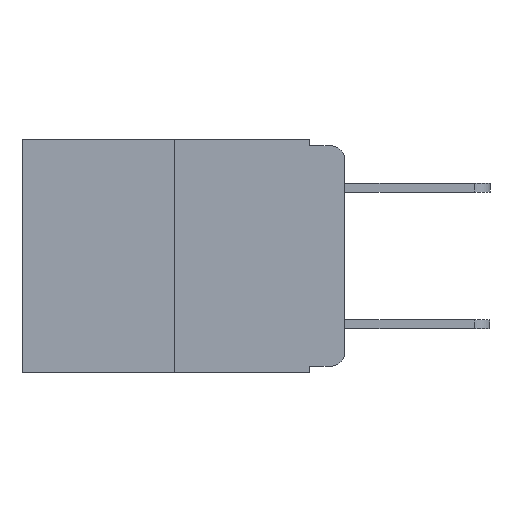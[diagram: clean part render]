
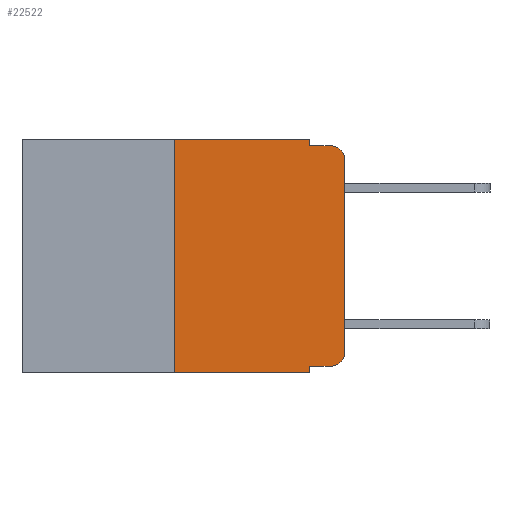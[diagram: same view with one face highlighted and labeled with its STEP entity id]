
A CAD part, left-side view. The second image highlights one B-rep face of the part: STEP entity #22522.
In plain terms, the highlighted planar face has unit normal (-1, 0, 0).
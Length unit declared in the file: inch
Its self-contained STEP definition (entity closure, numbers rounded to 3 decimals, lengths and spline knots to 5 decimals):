
#40 = ORIENTED_EDGE ( 'NONE', *, *, #12396, .T. ) ;
#79 = ORIENTED_EDGE ( 'NONE', *, *, #18576, .F. ) ;
#136 = DIRECTION ( 'NONE',  ( 0., 0., -1. ) ) ;
#841 = CIRCLE ( 'NONE', #1884, 0.02 ) ;
#1027 = ORIENTED_EDGE ( 'NONE', *, *, #13814, .F. ) ;
#1268 = CARTESIAN_POINT ( 'NONE',  ( 0., 0.25, -0.343 ) ) ;
#1884 = AXIS2_PLACEMENT_3D ( 'NONE', #23375, #11987, #136 ) ;
#2497 = DIRECTION ( 'NONE',  ( 0., 0., -1. ) ) ;
#2534 = CIRCLE ( 'NONE', #17583, 0.02 ) ;
#2597 = CARTESIAN_POINT ( 'NONE',  ( 0., 0.02, -0.313 ) ) ;
#2759 = VERTEX_POINT ( 'NONE', #7565 ) ;
#3263 = DIRECTION ( 'NONE',  ( 1., 0., 0. ) ) ;
#3293 = EDGE_LOOP ( 'NONE', ( #40, #3897, #21982, #24891, #1027, #79, #11259, #17466, #17170, #10684 ) ) ;
#3463 = CARTESIAN_POINT ( 'NONE',  ( 0., 0.051, -0.01 ) ) ;
#3897 = ORIENTED_EDGE ( 'NONE', *, *, #9848, .T. ) ;
#4304 = LINE ( 'NONE', #3463, #8917 ) ;
#4514 = EDGE_CURVE ( 'NONE', #22228, #10288, #9702, .T. ) ;
#4584 = DIRECTION ( 'NONE',  ( 0., 0., -1. ) ) ;
#6762 = LINE ( 'NONE', #21167, #16313 ) ;
#7042 = LINE ( 'NONE', #19482, #15984 ) ;
#7246 = EDGE_CURVE ( 'NONE', #10879, #13110, #19689, .T. ) ;
#7565 = CARTESIAN_POINT ( 'NONE',  ( 0., 0.02, -0.01 ) ) ;
#7959 = CARTESIAN_POINT ( 'NONE',  ( 0., 0.051, 0. ) ) ;
#8208 = CARTESIAN_POINT ( 'NONE',  ( 0., 0.051, -0.333 ) ) ;
#8228 = LINE ( 'NONE', #21622, #11248 ) ;
#8871 = VERTEX_POINT ( 'NONE', #13281 ) ;
#8917 = VECTOR ( 'NONE', #22626, 39.37008 ) ;
#9150 = EDGE_CURVE ( 'NONE', #8871, #21998, #2534, .T. ) ;
#9702 = LINE ( 'NONE', #15946, #17992 ) ;
#9848 = EDGE_CURVE ( 'NONE', #11433, #2759, #841, .T. ) ;
#9919 = DIRECTION ( 'NONE',  ( 0., 0., -1. ) ) ;
#9979 = DIRECTION ( 'NONE',  ( 0., -1., 0. ) ) ;
#10175 = DIRECTION ( 'NONE',  ( 0., -1., 0. ) ) ;
#10282 = CARTESIAN_POINT ( 'NONE',  ( 0., 0., -0.03 ) ) ;
#10288 = VERTEX_POINT ( 'NONE', #18878 ) ;
#10521 = VERTEX_POINT ( 'NONE', #19595 ) ;
#10684 = ORIENTED_EDGE ( 'NONE', *, *, #9150, .T. ) ;
#10819 = LINE ( 'NONE', #7959, #15815 ) ;
#10879 = VERTEX_POINT ( 'NONE', #1268 ) ;
#11248 = VECTOR ( 'NONE', #10175, 39.37008 ) ;
#11259 = ORIENTED_EDGE ( 'NONE', *, *, #7246, .T. ) ;
#11433 = VERTEX_POINT ( 'NONE', #10282 ) ;
#11514 = CARTESIAN_POINT ( 'NONE',  ( 0., 0.051, -0.343 ) ) ;
#11987 = DIRECTION ( 'NONE',  ( -1., 0., 0. ) ) ;
#12396 = EDGE_CURVE ( 'NONE', #21998, #11433, #6762, .T. ) ;
#12489 = EDGE_CURVE ( 'NONE', #10288, #2759, #4304, .T. ) ;
#13110 = VERTEX_POINT ( 'NONE', #11514 ) ;
#13281 = CARTESIAN_POINT ( 'NONE',  ( 0., 0.02, -0.333 ) ) ;
#13623 = CARTESIAN_POINT ( 'NONE',  ( 0., 0.25, 0. ) ) ;
#13814 = EDGE_CURVE ( 'NONE', #10521, #22228, #7042, .T. ) ;
#13967 = VECTOR ( 'NONE', #25031, 39.37008 ) ;
#14268 = FACE_OUTER_BOUND ( 'NONE', #3293, .T. ) ;
#14427 = AXIS2_PLACEMENT_3D ( 'NONE', #14795, #3263, #16723 ) ;
#14795 = CARTESIAN_POINT ( 'NONE',  ( 0., 0.473, 0. ) ) ;
#15255 = CARTESIAN_POINT ( 'NONE',  ( 0., 0., -0.313 ) ) ;
#15296 = EDGE_CURVE ( 'NONE', #18686, #8871, #8228, .T. ) ;
#15545 = DIRECTION ( 'NONE',  ( 0., -1., 0. ) ) ;
#15815 = VECTOR ( 'NONE', #9919, 39.37008 ) ;
#15946 = CARTESIAN_POINT ( 'NONE',  ( 0., 0.051, 0. ) ) ;
#15984 = VECTOR ( 'NONE', #9979, 39.37008 ) ;
#16069 = DIRECTION ( 'NONE',  ( -1., 0., 0. ) ) ;
#16313 = VECTOR ( 'NONE', #23074, 39.37008 ) ;
#16723 = DIRECTION ( 'NONE',  ( 0., 0., -1. ) ) ;
#17089 = EDGE_CURVE ( 'NONE', #18686, #13110, #10819, .T. ) ;
#17170 = ORIENTED_EDGE ( 'NONE', *, *, #15296, .T. ) ;
#17466 = ORIENTED_EDGE ( 'NONE', *, *, #17089, .F. ) ;
#17583 = AXIS2_PLACEMENT_3D ( 'NONE', #2597, #16069, #4584 ) ;
#17992 = VECTOR ( 'NONE', #2497, 39.37008 ) ;
#18576 = EDGE_CURVE ( 'NONE', #10879, #10521, #23524, .T. ) ;
#18686 = VERTEX_POINT ( 'NONE', #8208 ) ;
#18878 = CARTESIAN_POINT ( 'NONE',  ( 0., 0.051, -0.01 ) ) ;
#19482 = CARTESIAN_POINT ( 'NONE',  ( 0., 0.473, 0. ) ) ;
#19595 = CARTESIAN_POINT ( 'NONE',  ( 0., 0.25, 0. ) ) ;
#19689 = LINE ( 'NONE', #23180, #23296 ) ;
#21167 = CARTESIAN_POINT ( 'NONE',  ( 0., 0., 0. ) ) ;
#21622 = CARTESIAN_POINT ( 'NONE',  ( 0., 0.051, -0.333 ) ) ;
#21982 = ORIENTED_EDGE ( 'NONE', *, *, #12489, .F. ) ;
#21998 = VERTEX_POINT ( 'NONE', #15255 ) ;
#22228 = VERTEX_POINT ( 'NONE', #23427 ) ;
#22522 = ADVANCED_FACE ( 'NONE', ( #14268 ), #24312, .F. ) ;
#22626 = DIRECTION ( 'NONE',  ( 0., -1., 0. ) ) ;
#23074 = DIRECTION ( 'NONE',  ( 0., 0., 1. ) ) ;
#23180 = CARTESIAN_POINT ( 'NONE',  ( 0., 0.473, -0.343 ) ) ;
#23296 = VECTOR ( 'NONE', #15545, 39.37008 ) ;
#23375 = CARTESIAN_POINT ( 'NONE',  ( 0., 0.02, -0.03 ) ) ;
#23427 = CARTESIAN_POINT ( 'NONE',  ( 0., 0.051, 0. ) ) ;
#23524 = LINE ( 'NONE', #13623, #13967 ) ;
#24312 = PLANE ( 'NONE',  #14427 ) ;
#24891 = ORIENTED_EDGE ( 'NONE', *, *, #4514, .F. ) ;
#25031 = DIRECTION ( 'NONE',  ( 0., 0., 1. ) ) ;
